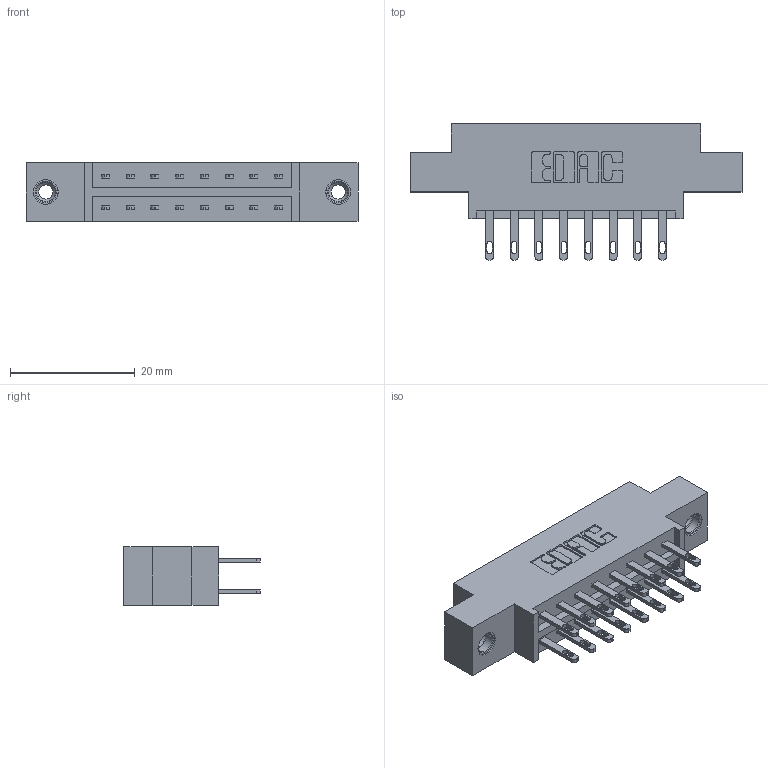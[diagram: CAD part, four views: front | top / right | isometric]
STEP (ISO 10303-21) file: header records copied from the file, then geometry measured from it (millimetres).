
FILE_DESCRIPTION (( 'STEP AP203' ), '1' );
FILE_NAME ('333-016-500-808.STEP', '2018-08-01T11:17:40', ( '' ), ( '' ), 'SwSTEP 2.0', 'SolidWorks 2016', '' );
FILE_SCHEMA (( 'CONFIG_CONTROL_DESIGN' ));
Length unit declared in the file: inch
Products named in the file (4): 345-250-001_345-250-003-102; 333-016-500-808; 333 Part_Offset - .156 Dia - TI; 345-292-001_345-293-100
Assembly tree (19 placements, depth 2):
  333-016-500-808
    333 Part_Offset - .156 Dia - TI
    345-292-001_345-293-100  x16
    345-250-001_345-250-003-102  x2
Bounding box: 53.24 x 21.85 x 9.4 mm (x, y, z)
Volume: 4932 mm3; surface area: 5884.1 mm2
Topology: 19 solids, 19 shells, 946 faces, 2811 edges, 1866 vertices
Faces by surface type: plane 586, cylinder 344, cone 12, torus 4
Entity records: 10792 total; most frequent: CARTESIAN_POINT 1813, ORIENTED_EDGE 1742, DIRECTION 1641, EDGE_CURVE 871, VECTOR 719, LINE 719, VERTEX_POINT 576, AXIS2_PLACEMENT_3D 461
